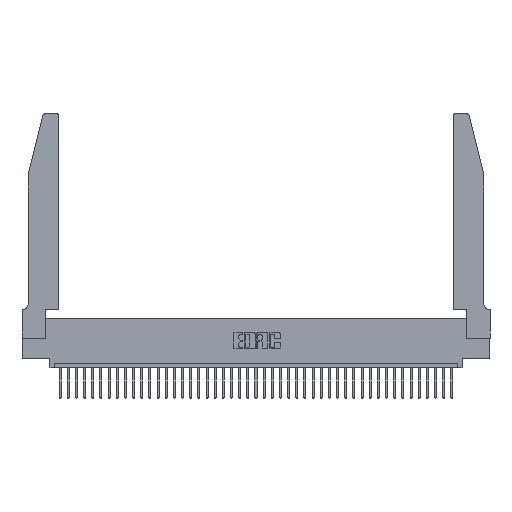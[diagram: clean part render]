
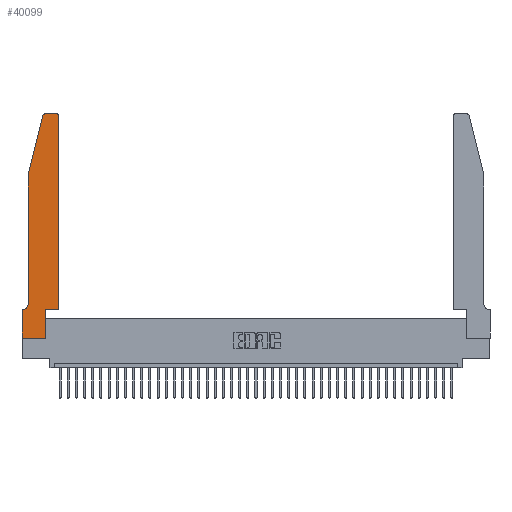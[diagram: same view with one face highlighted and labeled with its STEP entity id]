
A CAD part, top view. The second image highlights one B-rep face of the part: STEP entity #40099.
In plain terms, the highlighted planar face has unit normal (0, 0, 1).
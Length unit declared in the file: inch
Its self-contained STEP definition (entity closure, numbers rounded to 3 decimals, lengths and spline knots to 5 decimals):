
#25 = ORIENTED_EDGE ( 'NONE', *, *, #32198, .T. ) ;
#1348 = CARTESIAN_POINT ( 'NONE',  ( 0., 0.35, 0.37 ) ) ;
#1578 = CARTESIAN_POINT ( 'NONE',  ( 0.0055, 0.35, 0.37 ) ) ;
#1909 = VERTEX_POINT ( 'NONE', #31571 ) ;
#2244 = VERTEX_POINT ( 'NONE', #40405 ) ;
#2301 = CARTESIAN_POINT ( 'NONE',  ( 0.2865, 0.35, 0.37 ) ) ;
#3049 = CARTESIAN_POINT ( 'NONE',  ( 0.4505, 0.35, 0.37 ) ) ;
#3065 = AXIS2_PLACEMENT_3D ( 'NONE', #28062, #25014, #40647 ) ;
#3141 = VERTEX_POINT ( 'NONE', #11051 ) ;
#3594 = DIRECTION ( 'NONE',  ( 1., 0., 0. ) ) ;
#3610 = CARTESIAN_POINT ( 'NONE',  ( 0., 0., 0.37 ) ) ;
#3849 = DIRECTION ( 'NONE',  ( 0., -1., 0. ) ) ;
#3926 = CARTESIAN_POINT ( 'NONE',  ( 0.4205, 2.72, 0.37 ) ) ;
#3940 = EDGE_CURVE ( 'NONE', #3141, #17032, #36303, .T. ) ;
#4194 = VECTOR ( 'NONE', #15705, 39.37008 ) ;
#4894 = LINE ( 'NONE', #17321, #28104 ) ;
#5139 = ORIENTED_EDGE ( 'NONE', *, *, #33969, .T. ) ;
#5249 = EDGE_CURVE ( 'NONE', #17032, #25724, #22839, .T. ) ;
#5393 = ORIENTED_EDGE ( 'NONE', *, *, #32325, .T. ) ;
#6278 = EDGE_CURVE ( 'NONE', #32566, #15000, #8967, .T. ) ;
#6401 = FACE_OUTER_BOUND ( 'NONE', #31947, .T. ) ;
#6641 = LINE ( 'NONE', #3049, #19488 ) ;
#7084 = CARTESIAN_POINT ( 'NONE',  ( 0.4505, 0.35, 0.37 ) ) ;
#7338 = ORIENTED_EDGE ( 'NONE', *, *, #3940, .T. ) ;
#8871 = ORIENTED_EDGE ( 'NONE', *, *, #36359, .T. ) ;
#8967 = LINE ( 'NONE', #7084, #27163 ) ;
#9948 = CARTESIAN_POINT ( 'NONE',  ( 0.2865, 0.35, 0.37 ) ) ;
#10443 = CARTESIAN_POINT ( 'NONE',  ( 0.4505, 2.72, 0.37 ) ) ;
#11051 = CARTESIAN_POINT ( 'NONE',  ( 0.0755, 2., 0.37 ) ) ;
#11530 = CARTESIAN_POINT ( 'NONE',  ( 0.2865, 0., 0.37 ) ) ;
#11623 = VECTOR ( 'NONE', #38615, 39.37008 ) ;
#12060 = DIRECTION ( 'NONE',  ( 1., 0., 0. ) ) ;
#12164 = EDGE_CURVE ( 'NONE', #25724, #26447, #4894, .T. ) ;
#12279 = CARTESIAN_POINT ( 'NONE',  ( 0.2605, 2.75, 0.37 ) ) ;
#12487 = VERTEX_POINT ( 'NONE', #11530 ) ;
#12933 = DIRECTION ( 'NONE',  ( 0., 0., 1. ) ) ;
#14185 = LINE ( 'NONE', #22895, #39802 ) ;
#14491 = LINE ( 'NONE', #2301, #37668 ) ;
#15000 = VERTEX_POINT ( 'NONE', #10443 ) ;
#15705 = DIRECTION ( 'NONE',  ( 0., -1., 0. ) ) ;
#16041 = VECTOR ( 'NONE', #37669, 39.37008 ) ;
#16170 = EDGE_CURVE ( 'NONE', #21412, #2244, #37766, .T. ) ;
#16588 = PLANE ( 'NONE',  #24750 ) ;
#17032 = VERTEX_POINT ( 'NONE', #19783 ) ;
#17321 = CARTESIAN_POINT ( 'NONE',  ( 0.0755, 0.35, 0.37 ) ) ;
#19332 = DIRECTION ( 'NONE',  ( -1., 0., 0. ) ) ;
#19488 = VECTOR ( 'NONE', #12060, 39.37008 ) ;
#19566 = EDGE_CURVE ( 'NONE', #1909, #3141, #21248, .T. ) ;
#19712 = ORIENTED_EDGE ( 'NONE', *, *, #34544, .T. ) ;
#19783 = CARTESIAN_POINT ( 'NONE',  ( 0.0755, 0.42, 0.37 ) ) ;
#20011 = CARTESIAN_POINT ( 'NONE',  ( 0.4505, 0.35, 0.37 ) ) ;
#20020 = LINE ( 'NONE', #37584, #11623 ) ;
#20041 = CARTESIAN_POINT ( 'NONE',  ( 0.284, 2.72, 0.37 ) ) ;
#20684 = CARTESIAN_POINT ( 'NONE',  ( 0.4205, 2.75, 0.37 ) ) ;
#21248 = LINE ( 'NONE', #23213, #29534 ) ;
#21412 = VERTEX_POINT ( 'NONE', #20684 ) ;
#22241 = DIRECTION ( 'NONE',  ( 0., 0., 1. ) ) ;
#22833 = DIRECTION ( 'NONE',  ( 1., 0., 0. ) ) ;
#22839 = CIRCLE ( 'NONE', #3065, 0.07 ) ;
#22895 = CARTESIAN_POINT ( 'NONE',  ( 0., 0., 0.37 ) ) ;
#23213 = CARTESIAN_POINT ( 'NONE',  ( 0.0755, 2., 0.37 ) ) ;
#23348 = DIRECTION ( 'NONE',  ( 0., 1., 0. ) ) ;
#23626 = DIRECTION ( 'NONE',  ( -0.239, -0.971, 0. ) ) ;
#24750 = AXIS2_PLACEMENT_3D ( 'NONE', #28818, #22241, #3594 ) ;
#25014 = DIRECTION ( 'NONE',  ( 0., 0., -1. ) ) ;
#25724 = VERTEX_POINT ( 'NONE', #1578 ) ;
#26151 = DIRECTION ( 'NONE',  ( 1., 0., 0. ) ) ;
#26447 = VERTEX_POINT ( 'NONE', #1348 ) ;
#27163 = VECTOR ( 'NONE', #23348, 39.37008 ) ;
#28062 = CARTESIAN_POINT ( 'NONE',  ( 0.0055, 0.42, 0.37 ) ) ;
#28104 = VECTOR ( 'NONE', #19332, 39.37008 ) ;
#28818 = CARTESIAN_POINT ( 'NONE',  ( 0., 0.35, 0.37 ) ) ;
#29008 = ORIENTED_EDGE ( 'NONE', *, *, #6278, .T. ) ;
#29534 = VECTOR ( 'NONE', #23626, 39.37008 ) ;
#31252 = CIRCLE ( 'NONE', #36267, 0.03 ) ;
#31571 = CARTESIAN_POINT ( 'NONE',  ( 0.25487, 2.72718, 0.37 ) ) ;
#31947 = EDGE_LOOP ( 'NONE', ( #36963, #38688, #34403, #7338, #40851, #35234, #8871, #25, #19712, #5393, #29008, #5139 ) ) ;
#32198 = EDGE_CURVE ( 'NONE', #33450, #12487, #20020, .T. ) ;
#32325 = EDGE_CURVE ( 'NONE', #35970, #32566, #6641, .T. ) ;
#32534 = DIRECTION ( 'NONE',  ( 0., 0., 1. ) ) ;
#32566 = VERTEX_POINT ( 'NONE', #20011 ) ;
#33450 = VERTEX_POINT ( 'NONE', #3610 ) ;
#33969 = EDGE_CURVE ( 'NONE', #15000, #21412, #31252, .T. ) ;
#34403 = ORIENTED_EDGE ( 'NONE', *, *, #19566, .T. ) ;
#34544 = EDGE_CURVE ( 'NONE', #12487, #35970, #14491, .T. ) ;
#34578 = CARTESIAN_POINT ( 'NONE',  ( 0.0755, 2., 0.37 ) ) ;
#35234 = ORIENTED_EDGE ( 'NONE', *, *, #12164, .T. ) ;
#35970 = VERTEX_POINT ( 'NONE', #9948 ) ;
#36267 = AXIS2_PLACEMENT_3D ( 'NONE', #3926, #12933, #22833 ) ;
#36303 = LINE ( 'NONE', #34578, #4194 ) ;
#36359 = EDGE_CURVE ( 'NONE', #26447, #33450, #14185, .T. ) ;
#36440 = EDGE_CURVE ( 'NONE', #2244, #1909, #37394, .T. ) ;
#36963 = ORIENTED_EDGE ( 'NONE', *, *, #16170, .T. ) ;
#37394 = CIRCLE ( 'NONE', #39455, 0.03 ) ;
#37584 = CARTESIAN_POINT ( 'NONE',  ( 0., 0., 0.37 ) ) ;
#37668 = VECTOR ( 'NONE', #40638, 39.37008 ) ;
#37669 = DIRECTION ( 'NONE',  ( -1., 0., 0. ) ) ;
#37766 = LINE ( 'NONE', #12279, #16041 ) ;
#38615 = DIRECTION ( 'NONE',  ( 1., 0., 0. ) ) ;
#38688 = ORIENTED_EDGE ( 'NONE', *, *, #36440, .T. ) ;
#39455 = AXIS2_PLACEMENT_3D ( 'NONE', #20041, #32534, #26151 ) ;
#39802 = VECTOR ( 'NONE', #3849, 39.37008 ) ;
#40099 = ADVANCED_FACE ( 'NONE', ( #6401 ), #16588, .T. ) ;
#40405 = CARTESIAN_POINT ( 'NONE',  ( 0.284, 2.75, 0.37 ) ) ;
#40638 = DIRECTION ( 'NONE',  ( 0., 1., 0. ) ) ;
#40647 = DIRECTION ( 'NONE',  ( -1., 0., 0. ) ) ;
#40851 = ORIENTED_EDGE ( 'NONE', *, *, #5249, .T. ) ;
